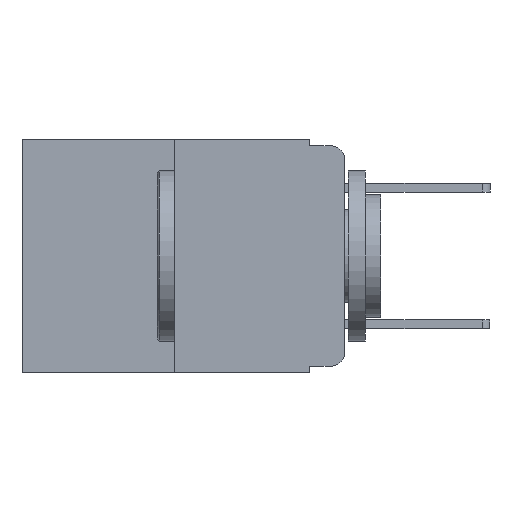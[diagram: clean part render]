
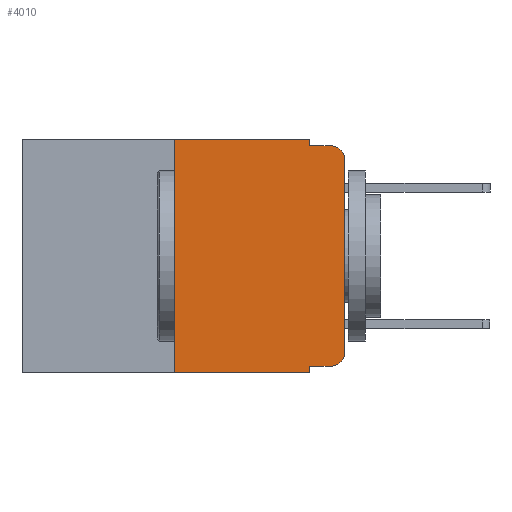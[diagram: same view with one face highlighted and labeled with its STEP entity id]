
A CAD part, left-side view. The second image highlights one B-rep face of the part: STEP entity #4010.
In plain terms, the highlighted planar face has unit normal (-1, 0, 0).
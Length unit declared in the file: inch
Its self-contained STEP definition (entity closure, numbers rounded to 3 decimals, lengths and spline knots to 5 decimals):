
#76 = EDGE_CURVE ( 'NONE', #10701, #2656, #4369, .T. ) ;
#205 = ORIENTED_EDGE ( 'NONE', *, *, #6232, .T. ) ;
#410 = LINE ( 'NONE', #2098, #4365 ) ;
#452 = DIRECTION ( 'NONE',  ( 0., 0., -1. ) ) ;
#490 = DIRECTION ( 'NONE',  ( -1., 0., 0. ) ) ;
#619 = VERTEX_POINT ( 'NONE', #3793 ) ;
#749 = EDGE_LOOP ( 'NONE', ( #3652, #4614, #1307, #7314, #10898, #2941, #205, #7708, #5539, #16215 ) ) ;
#828 = VERTEX_POINT ( 'NONE', #2957 ) ;
#863 = AXIS2_PLACEMENT_3D ( 'NONE', #14106, #14034, #2361 ) ;
#930 = CARTESIAN_POINT ( 'NONE',  ( 0., 0.051, 0. ) ) ;
#1195 = CARTESIAN_POINT ( 'NONE',  ( 0., 0.02, -0.333 ) ) ;
#1307 = ORIENTED_EDGE ( 'NONE', *, *, #5486, .F. ) ;
#1745 = CARTESIAN_POINT ( 'NONE',  ( 0., 0.02, -0.313 ) ) ;
#1860 = VERTEX_POINT ( 'NONE', #10206 ) ;
#2006 = LINE ( 'NONE', #11912, #5542 ) ;
#2098 = CARTESIAN_POINT ( 'NONE',  ( 0., 0.473, -0.343 ) ) ;
#2137 = DIRECTION ( 'NONE',  ( 0., -1., 0. ) ) ;
#2212 = VERTEX_POINT ( 'NONE', #930 ) ;
#2361 = DIRECTION ( 'NONE',  ( 0., 0., -1. ) ) ;
#2398 = CIRCLE ( 'NONE', #6961, 0.02 ) ;
#2527 = LINE ( 'NONE', #2861, #12430 ) ;
#2656 = VERTEX_POINT ( 'NONE', #9489 ) ;
#2861 = CARTESIAN_POINT ( 'NONE',  ( 0., 0.25, 0. ) ) ;
#2941 = ORIENTED_EDGE ( 'NONE', *, *, #13006, .F. ) ;
#2949 = CARTESIAN_POINT ( 'NONE',  ( 0., 0.25, -0.343 ) ) ;
#2957 = CARTESIAN_POINT ( 'NONE',  ( 0., 0.02, -0.01 ) ) ;
#3245 = CARTESIAN_POINT ( 'NONE',  ( 0., 0., 0. ) ) ;
#3485 = DIRECTION ( 'NONE',  ( -1., 0., 0. ) ) ;
#3652 = ORIENTED_EDGE ( 'NONE', *, *, #76, .T. ) ;
#3778 = CARTESIAN_POINT ( 'NONE',  ( 0., 0.051, -0.01 ) ) ;
#3793 = CARTESIAN_POINT ( 'NONE',  ( 0., 0.25, 0. ) ) ;
#4010 = ADVANCED_FACE ( 'NONE', ( #5413 ), #15712, .F. ) ;
#4144 = CARTESIAN_POINT ( 'NONE',  ( 0., 0.051, -0.343 ) ) ;
#4269 = AXIS2_PLACEMENT_3D ( 'NONE', #1745, #490, #452 ) ;
#4345 = EDGE_CURVE ( 'NONE', #619, #2212, #10432, .T. ) ;
#4365 = VECTOR ( 'NONE', #2137, 39.37008 ) ;
#4369 = LINE ( 'NONE', #3245, #13838 ) ;
#4614 = ORIENTED_EDGE ( 'NONE', *, *, #8025, .T. ) ;
#5019 = EDGE_CURVE ( 'NONE', #9069, #10701, #8318, .T. ) ;
#5413 = FACE_OUTER_BOUND ( 'NONE', #749, .T. ) ;
#5486 = EDGE_CURVE ( 'NONE', #12805, #828, #15874, .T. ) ;
#5532 = DIRECTION ( 'NONE',  ( 0., -1., 0. ) ) ;
#5539 = ORIENTED_EDGE ( 'NONE', *, *, #6406, .T. ) ;
#5542 = VECTOR ( 'NONE', #13095, 39.37008 ) ;
#5727 = CARTESIAN_POINT ( 'NONE',  ( 0., 0.051, -0.333 ) ) ;
#5849 = DIRECTION ( 'NONE',  ( 0., 0., 1. ) ) ;
#6134 = CARTESIAN_POINT ( 'NONE',  ( 0., 0., -0.313 ) ) ;
#6232 = EDGE_CURVE ( 'NONE', #8532, #14570, #410, .T. ) ;
#6406 = EDGE_CURVE ( 'NONE', #1860, #9069, #10702, .T. ) ;
#6813 = CARTESIAN_POINT ( 'NONE',  ( 0., 0.051, -0.01 ) ) ;
#6900 = DIRECTION ( 'NONE',  ( 0., 0., -1. ) ) ;
#6961 = AXIS2_PLACEMENT_3D ( 'NONE', #11202, #3485, #12393 ) ;
#7314 = ORIENTED_EDGE ( 'NONE', *, *, #14672, .F. ) ;
#7501 = VECTOR ( 'NONE', #5532, 39.37008 ) ;
#7546 = EDGE_CURVE ( 'NONE', #1860, #14570, #9927, .T. ) ;
#7708 = ORIENTED_EDGE ( 'NONE', *, *, #7546, .F. ) ;
#8003 = DIRECTION ( 'NONE',  ( 0., -1., 0. ) ) ;
#8025 = EDGE_CURVE ( 'NONE', #2656, #828, #2398, .T. ) ;
#8318 = CIRCLE ( 'NONE', #4269, 0.02 ) ;
#8532 = VERTEX_POINT ( 'NONE', #2949 ) ;
#9069 = VERTEX_POINT ( 'NONE', #1195 ) ;
#9489 = CARTESIAN_POINT ( 'NONE',  ( 0., 0., -0.03 ) ) ;
#9505 = DIRECTION ( 'NONE',  ( 0., 0., 1. ) ) ;
#9927 = LINE ( 'NONE', #16360, #15053 ) ;
#10206 = CARTESIAN_POINT ( 'NONE',  ( 0., 0.051, -0.333 ) ) ;
#10432 = LINE ( 'NONE', #12363, #13184 ) ;
#10701 = VERTEX_POINT ( 'NONE', #6134 ) ;
#10702 = LINE ( 'NONE', #5727, #7501 ) ;
#10898 = ORIENTED_EDGE ( 'NONE', *, *, #4345, .F. ) ;
#11202 = CARTESIAN_POINT ( 'NONE',  ( 0., 0.02, -0.03 ) ) ;
#11912 = CARTESIAN_POINT ( 'NONE',  ( 0., 0.051, 0. ) ) ;
#12363 = CARTESIAN_POINT ( 'NONE',  ( 0., 0.473, 0. ) ) ;
#12393 = DIRECTION ( 'NONE',  ( 0., 0., -1. ) ) ;
#12430 = VECTOR ( 'NONE', #5849, 39.37008 ) ;
#12782 = VECTOR ( 'NONE', #8003, 39.37008 ) ;
#12805 = VERTEX_POINT ( 'NONE', #6813 ) ;
#13006 = EDGE_CURVE ( 'NONE', #8532, #619, #2527, .T. ) ;
#13095 = DIRECTION ( 'NONE',  ( 0., 0., -1. ) ) ;
#13184 = VECTOR ( 'NONE', #16165, 39.37008 ) ;
#13838 = VECTOR ( 'NONE', #9505, 39.37008 ) ;
#14034 = DIRECTION ( 'NONE',  ( 1., 0., 0. ) ) ;
#14106 = CARTESIAN_POINT ( 'NONE',  ( 0., 0.473, 0. ) ) ;
#14570 = VERTEX_POINT ( 'NONE', #4144 ) ;
#14672 = EDGE_CURVE ( 'NONE', #2212, #12805, #2006, .T. ) ;
#15053 = VECTOR ( 'NONE', #6900, 39.37008 ) ;
#15712 = PLANE ( 'NONE',  #863 ) ;
#15874 = LINE ( 'NONE', #3778, #12782 ) ;
#16165 = DIRECTION ( 'NONE',  ( 0., -1., 0. ) ) ;
#16215 = ORIENTED_EDGE ( 'NONE', *, *, #5019, .T. ) ;
#16360 = CARTESIAN_POINT ( 'NONE',  ( 0., 0.051, 0. ) ) ;
